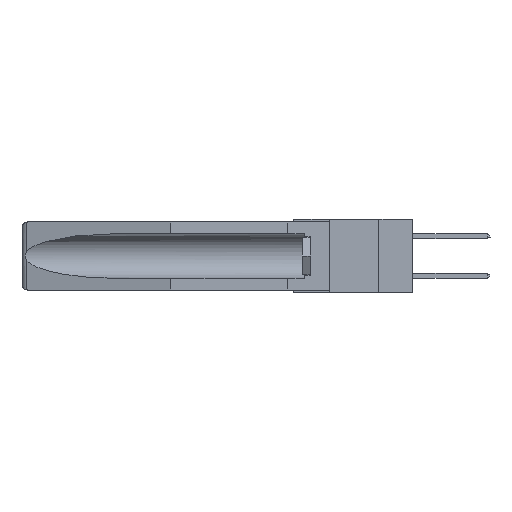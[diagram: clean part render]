
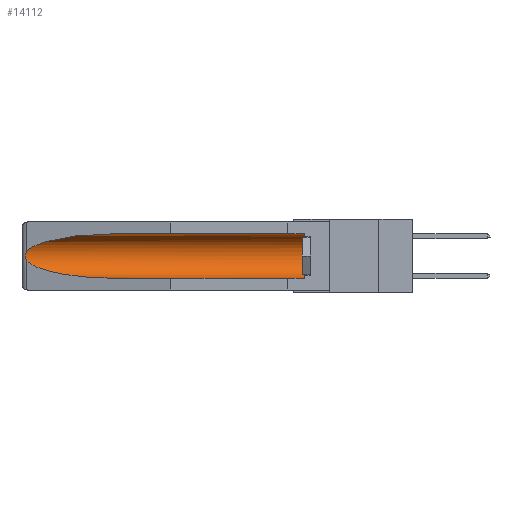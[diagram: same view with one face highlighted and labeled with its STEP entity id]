
A CAD part, left-side view. The second image highlights one B-rep face of the part: STEP entity #14112.
In plain terms, the highlighted cylindrical face has radius 2.857 mm (diameter 5.715 mm), a partial arc.
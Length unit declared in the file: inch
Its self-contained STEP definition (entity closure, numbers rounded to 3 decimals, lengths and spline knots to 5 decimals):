
#359 = CARTESIAN_POINT ( 'NONE',  ( 0.155, 1.07973, -0.059 ) ) ;
#1134 = CARTESIAN_POINT ( 'NONE',  ( 0.2673, 1.53269, -0.17917 ) ) ;
#1776 = CARTESIAN_POINT ( 'NONE',  ( 0.155, 0.126, -0.1715 ) ) ;
#2192 = EDGE_CURVE ( 'NONE', #12235, #28557, #28750, .T. ) ;
#2483 = CARTESIAN_POINT ( 'NONE',  ( 0.26537, 1.52718, -0.19328 ) ) ;
#2854 = B_SPLINE_CURVE_WITH_KNOTS ( 'NONE', 3,
 ( #28954, #15014, #5870, #24245, #22081, #15115, #1134, #17151, #8224, #10547 ),
 .UNSPECIFIED., .F., .F.,
 ( 4, 2, 2, 2, 4 ),
 ( 0., 0.00029, 0.00058, 0.00087, 0.00117 ),
 .UNSPECIFIED. ) ;
#3955 = VERTEX_POINT ( 'NONE', #2483 ) ;
#4519 = ORIENTED_EDGE ( 'NONE', *, *, #12430, .T. ) ;
#5087 = CARTESIAN_POINT ( 'NONE',  ( 0.21114, 1.30732, -0.059 ) ) ;
#5870 = CARTESIAN_POINT ( 'NONE',  ( 0.26654, 1.53092, -0.15636 ) ) ;
#7578 = CARTESIAN_POINT ( 'NONE',  ( 0.155, 1.07973, -0.059 ) ) ;
#7829 = CARTESIAN_POINT ( 'NONE',  ( 0.26537, 1.52718, -0.14972 ) ) ;
#8212 = VERTEX_POINT ( 'NONE', #7578 ) ;
#8224 = CARTESIAN_POINT ( 'NONE',  ( 0.26597, 1.5296, -0.19026 ) ) ;
#10279 = CARTESIAN_POINT ( 'NONE',  ( 0.155, 1.07973, -0.284 ) ) ;
#10388 = EDGE_CURVE ( 'NONE', #12235, #14649, #24250, .T. ) ;
#10547 = CARTESIAN_POINT ( 'NONE',  ( 0.26537, 1.52718, -0.19328 ) ) ;
#10911 = CARTESIAN_POINT ( 'NONE',  ( 0.155, 0.126, -0.284 ) ) ;
#11039 = DIRECTION ( 'NONE',  ( 0., 1., 0. ) ) ;
#11090 = DIRECTION ( 'NONE',  ( 0., -1., 0. ) ) ;
#11342 = EDGE_CURVE ( 'NONE', #3955, #28557, #13063, .T. ) ;
#11658 = DIRECTION ( 'NONE',  ( 0., 1., 0. ) ) ;
#12235 = VERTEX_POINT ( 'NONE', #10911 ) ;
#12284 = VECTOR ( 'NONE', #11039, 39.37008 ) ;
#12430 = EDGE_CURVE ( 'NONE', #14649, #8212, #24597, .T. ) ;
#13063 =( BOUNDED_CURVE ( )  B_SPLINE_CURVE ( 3, ( #18418, #16202, #20968, #22977 ),
 .UNSPECIFIED., .F., .F. ) 
 B_SPLINE_CURVE_WITH_KNOTS ( ( 4, 4 ),
 ( 0.1948, 1.5708 ),
 .UNSPECIFIED. ) 
 CURVE ( )  GEOMETRIC_REPRESENTATION_ITEM ( )  RATIONAL_B_SPLINE_CURVE ( ( 1., 0.848, 0.848, 1. ) ) 
 REPRESENTATION_ITEM ( '' )  );
#13229 = CARTESIAN_POINT ( 'NONE',  ( 0.155, 0.126, -0.059 ) ) ;
#13609 = CARTESIAN_POINT ( 'NONE',  ( 0.155, -0.30754, -0.284 ) ) ;
#13834 = ORIENTED_EDGE ( 'NONE', *, *, #22396, .T. ) ;
#13977 = VECTOR ( 'NONE', #20671, 39.37008 ) ;
#14015 = AXIS2_PLACEMENT_3D ( 'NONE', #1776, #11090, #27271 ) ;
#14112 = ADVANCED_FACE ( 'NONE', ( #29528 ), #21562, .F. ) ;
#14649 = VERTEX_POINT ( 'NONE', #13229 ) ;
#15014 = CARTESIAN_POINT ( 'NONE',  ( 0.26597, 1.52961, -0.15275 ) ) ;
#15115 = CARTESIAN_POINT ( 'NONE',  ( 0.2675, 1.53308, -0.17534 ) ) ;
#15254 = ORIENTED_EDGE ( 'NONE', *, *, #29234, .T. ) ;
#15557 = CARTESIAN_POINT ( 'NONE',  ( 0.26537, 1.52718, -0.14972 ) ) ;
#15804 = CARTESIAN_POINT ( 'NONE',  ( 0.155, -0.30754, -0.1715 ) ) ;
#16202 = CARTESIAN_POINT ( 'NONE',  ( 0.25451, 1.48313, -0.24835 ) ) ;
#16458 = EDGE_LOOP ( 'NONE', ( #13834, #15254, #26561, #29551, #16930, #4519 ) ) ;
#16842 = CARTESIAN_POINT ( 'NONE',  ( 0.155, -0.30754, -0.059 ) ) ;
#16930 = ORIENTED_EDGE ( 'NONE', *, *, #10388, .T. ) ;
#16955 = CARTESIAN_POINT ( 'NONE',  ( 0.25451, 1.48313, -0.09465 ) ) ;
#17151 = CARTESIAN_POINT ( 'NONE',  ( 0.26655, 1.53094, -0.18657 ) ) ;
#18418 = CARTESIAN_POINT ( 'NONE',  ( 0.26537, 1.52718, -0.19328 ) ) ;
#20671 = DIRECTION ( 'NONE',  ( 0., 1., 0. ) ) ;
#20968 = CARTESIAN_POINT ( 'NONE',  ( 0.21114, 1.30732, -0.284 ) ) ;
#21562 = CYLINDRICAL_SURFACE ( 'NONE', #21987, 0.1125 ) ;
#21987 = AXIS2_PLACEMENT_3D ( 'NONE', #15804, #11658, #27820 ) ;
#22057 = VERTEX_POINT ( 'NONE', #15557 ) ;
#22081 = CARTESIAN_POINT ( 'NONE',  ( 0.2675, 1.53308, -0.16763 ) ) ;
#22396 = EDGE_CURVE ( 'NONE', #8212, #22057, #28989, .T. ) ;
#22977 = CARTESIAN_POINT ( 'NONE',  ( 0.155, 1.07973, -0.284 ) ) ;
#24245 = CARTESIAN_POINT ( 'NONE',  ( 0.2673, 1.5327, -0.16383 ) ) ;
#24250 = CIRCLE ( 'NONE', #14015, 0.1125 ) ;
#24597 = LINE ( 'NONE', #16842, #12284 ) ;
#26561 = ORIENTED_EDGE ( 'NONE', *, *, #11342, .T. ) ;
#27271 = DIRECTION ( 'NONE',  ( 0., 0., 1. ) ) ;
#27820 = DIRECTION ( 'NONE',  ( 0., 0., 1. ) ) ;
#28557 = VERTEX_POINT ( 'NONE', #10279 ) ;
#28750 = LINE ( 'NONE', #13609, #13977 ) ;
#28954 = CARTESIAN_POINT ( 'NONE',  ( 0.26537, 1.52718, -0.14972 ) ) ;
#28989 =( BOUNDED_CURVE ( )  B_SPLINE_CURVE ( 3, ( #359, #5087, #16955, #7829 ),
 .UNSPECIFIED., .F., .T. ) 
 B_SPLINE_CURVE_WITH_KNOTS ( ( 4, 4 ),
 ( 4.71239, 6.08839 ),
 .UNSPECIFIED. ) 
 CURVE ( )  GEOMETRIC_REPRESENTATION_ITEM ( )  RATIONAL_B_SPLINE_CURVE ( ( 1., 0.848, 0.848, 1. ) ) 
 REPRESENTATION_ITEM ( '' )  );
#29234 = EDGE_CURVE ( 'NONE', #22057, #3955, #2854, .T. ) ;
#29528 = FACE_OUTER_BOUND ( 'NONE', #16458, .T. ) ;
#29551 = ORIENTED_EDGE ( 'NONE', *, *, #2192, .F. ) ;
